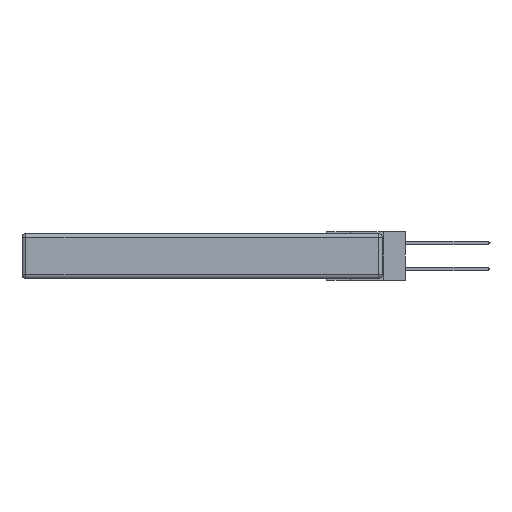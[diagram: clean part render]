
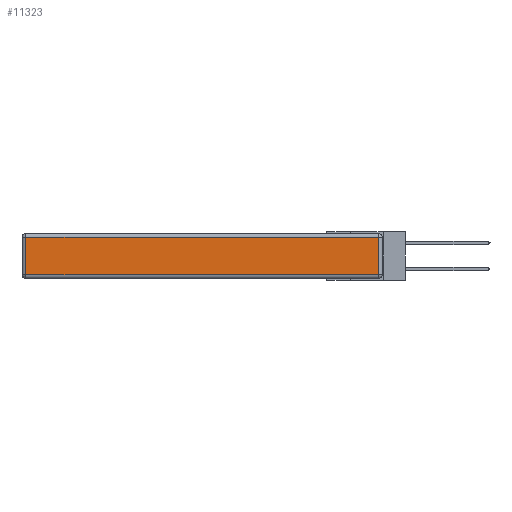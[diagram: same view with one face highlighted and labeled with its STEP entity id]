
A CAD part, left-side view. The second image highlights one B-rep face of the part: STEP entity #11323.
In plain terms, the highlighted planar face has unit normal (-1, 0, 0).
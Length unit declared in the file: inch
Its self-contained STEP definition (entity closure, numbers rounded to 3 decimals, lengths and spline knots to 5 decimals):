
#974 = DIRECTION ( 'NONE',  ( 0., 0., 1. ) ) ;
#2280 = ORIENTED_EDGE ( 'NONE', *, *, #19795, .T. ) ;
#2912 = VECTOR ( 'NONE', #29826, 39.37008 ) ;
#2931 = FACE_OUTER_BOUND ( 'NONE', #7072, .T. ) ;
#4124 = CARTESIAN_POINT ( 'NONE',  ( 0., 2.72, -0.313 ) ) ;
#4460 = LINE ( 'NONE', #30053, #2912 ) ;
#4897 = EDGE_CURVE ( 'NONE', #17669, #27600, #31904, .T. ) ;
#5155 = VERTEX_POINT ( 'NONE', #27426 ) ;
#7072 = EDGE_LOOP ( 'NONE', ( #27273, #28969, #2280, #25649 ) ) ;
#8076 = CARTESIAN_POINT ( 'NONE',  ( 0., 0.03, -0.03 ) ) ;
#9049 = DIRECTION ( 'NONE',  ( 0., 0., -1. ) ) ;
#11323 = ADVANCED_FACE ( 'NONE', ( #2931 ), #21060, .T. ) ;
#11460 = AXIS2_PLACEMENT_3D ( 'NONE', #15709, #16030, #974 ) ;
#13080 = LINE ( 'NONE', #20047, #20858 ) ;
#13186 = CARTESIAN_POINT ( 'NONE',  ( 0., 0.03, -0.313 ) ) ;
#13336 = CARTESIAN_POINT ( 'NONE',  ( 0., 0., -0.313 ) ) ;
#13429 = LINE ( 'NONE', #21519, #25913 ) ;
#13809 = EDGE_CURVE ( 'NONE', #27600, #15538, #4460, .T. ) ;
#15538 = VERTEX_POINT ( 'NONE', #8076 ) ;
#15709 = CARTESIAN_POINT ( 'NONE',  ( 0., 0., -0.343 ) ) ;
#16030 = DIRECTION ( 'NONE',  ( -1., 0., 0. ) ) ;
#17669 = VERTEX_POINT ( 'NONE', #4124 ) ;
#18366 = DIRECTION ( 'NONE',  ( 0., -1., 0. ) ) ;
#19795 = EDGE_CURVE ( 'NONE', #15538, #5155, #13080, .T. ) ;
#20047 = CARTESIAN_POINT ( 'NONE',  ( 0., 2.75, -0.03 ) ) ;
#20604 = EDGE_CURVE ( 'NONE', #5155, #17669, #13429, .T. ) ;
#20858 = VECTOR ( 'NONE', #24630, 39.37008 ) ;
#21060 = PLANE ( 'NONE',  #11460 ) ;
#21519 = CARTESIAN_POINT ( 'NONE',  ( 0., 2.72, -0.343 ) ) ;
#24630 = DIRECTION ( 'NONE',  ( 0., 1., 0. ) ) ;
#25649 = ORIENTED_EDGE ( 'NONE', *, *, #20604, .T. ) ;
#25913 = VECTOR ( 'NONE', #9049, 39.37008 ) ;
#27273 = ORIENTED_EDGE ( 'NONE', *, *, #4897, .T. ) ;
#27426 = CARTESIAN_POINT ( 'NONE',  ( 0., 2.72, -0.03 ) ) ;
#27600 = VERTEX_POINT ( 'NONE', #13186 ) ;
#28969 = ORIENTED_EDGE ( 'NONE', *, *, #13809, .T. ) ;
#29186 = VECTOR ( 'NONE', #18366, 39.37008 ) ;
#29826 = DIRECTION ( 'NONE',  ( 0., 0., 1. ) ) ;
#30053 = CARTESIAN_POINT ( 'NONE',  ( 0., 0.03, -0.343 ) ) ;
#31904 = LINE ( 'NONE', #13336, #29186 ) ;
